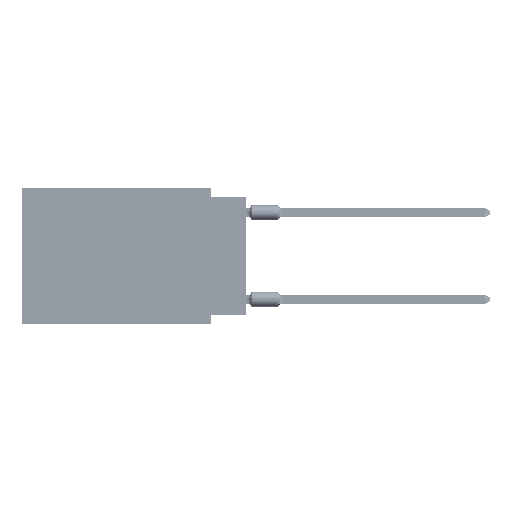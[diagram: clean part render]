
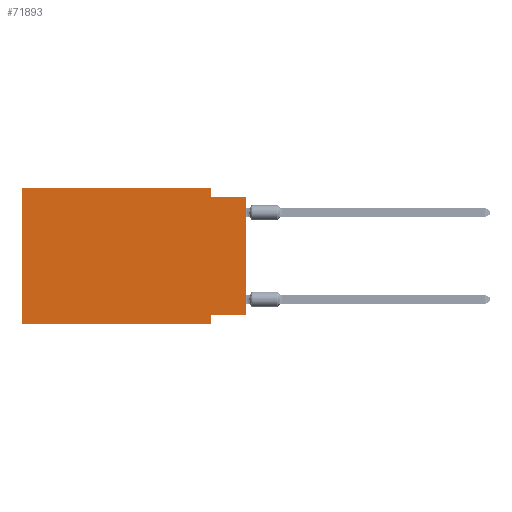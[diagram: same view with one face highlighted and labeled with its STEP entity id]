
A CAD part, left-side view. The second image highlights one B-rep face of the part: STEP entity #71893.
In plain terms, the highlighted planar face has unit normal (-1, 0, 0).
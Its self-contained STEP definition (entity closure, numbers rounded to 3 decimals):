
#214 = CARTESIAN_POINT ( 'NONE',  ( 0., 16.383, 0. ) ) ;
#407 = CARTESIAN_POINT ( 'NONE',  ( 0., 16.383, -9.906 ) ) ;
#1781 = LINE ( 'NONE', #71498, #9529 ) ;
#2015 = LINE ( 'NONE', #15659, #51012 ) ;
#5107 = EDGE_CURVE ( 'NONE', #33575, #48705, #1781, .T. ) ;
#5510 = CARTESIAN_POINT ( 'NONE',  ( 0., 16.383, 0. ) ) ;
#5823 = DIRECTION ( 'NONE',  ( 1., 0., 0. ) ) ;
#6408 = CARTESIAN_POINT ( 'NONE',  ( 0., 0., -0.635 ) ) ;
#9487 = DIRECTION ( 'NONE',  ( 0., 0., 1. ) ) ;
#9529 = VECTOR ( 'NONE', #23167, 1000. ) ;
#9564 = ORIENTED_EDGE ( 'NONE', *, *, #29825, .F. ) ;
#10591 = VERTEX_POINT ( 'NONE', #35574 ) ;
#11127 = VECTOR ( 'NONE', #9487, 1000. ) ;
#11436 = DIRECTION ( 'NONE',  ( 0., -1., 0. ) ) ;
#12645 = FACE_OUTER_BOUND ( 'NONE', #25397, .T. ) ;
#12924 = CARTESIAN_POINT ( 'NONE',  ( 0., 2.54, -9.906 ) ) ;
#15659 = CARTESIAN_POINT ( 'NONE',  ( 0., 0., -0.635 ) ) ;
#19621 = DIRECTION ( 'NONE',  ( 0., -1., 0. ) ) ;
#20076 = ORIENTED_EDGE ( 'NONE', *, *, #5107, .F. ) ;
#21809 = CARTESIAN_POINT ( 'NONE',  ( 0., 2.54, -9.271 ) ) ;
#22776 = EDGE_CURVE ( 'NONE', #80145, #86815, #71934, .T. ) ;
#23085 = CARTESIAN_POINT ( 'NONE',  ( 0., 0., -9.271 ) ) ;
#23167 = DIRECTION ( 'NONE',  ( 0., 0., -1. ) ) ;
#24443 = LINE ( 'NONE', #23085, #74344 ) ;
#25397 = EDGE_LOOP ( 'NONE', ( #33889, #69377, #9564, #27735, #79737, #35494, #20076, #78307 ) ) ;
#25433 = VECTOR ( 'NONE', #43156, 1000. ) ;
#27735 = ORIENTED_EDGE ( 'NONE', *, *, #51779, .F. ) ;
#29825 = EDGE_CURVE ( 'NONE', #10591, #76519, #44057, .T. ) ;
#31224 = VERTEX_POINT ( 'NONE', #407 ) ;
#31900 = VECTOR ( 'NONE', #11436, 1000. ) ;
#33575 = VERTEX_POINT ( 'NONE', #21809 ) ;
#33889 = ORIENTED_EDGE ( 'NONE', *, *, #22776, .T. ) ;
#33944 = AXIS2_PLACEMENT_3D ( 'NONE', #68262, #5823, #79807 ) ;
#35494 = ORIENTED_EDGE ( 'NONE', *, *, #82817, .T. ) ;
#35574 = CARTESIAN_POINT ( 'NONE',  ( 0., 2.54, 0. ) ) ;
#37668 = DIRECTION ( 'NONE',  ( 0., 1., 0. ) ) ;
#38788 = CARTESIAN_POINT ( 'NONE',  ( 0., 16.383, -9.906 ) ) ;
#40441 = PLANE ( 'NONE',  #33944 ) ;
#40640 = CARTESIAN_POINT ( 'NONE',  ( 0., 0., -9.271 ) ) ;
#43156 = DIRECTION ( 'NONE',  ( 0., 0., -1. ) ) ;
#44057 = LINE ( 'NONE', #85517, #25433 ) ;
#45671 = VECTOR ( 'NONE', #79933, 1000. ) ;
#48705 = VERTEX_POINT ( 'NONE', #12924 ) ;
#49818 = EDGE_CURVE ( 'NONE', #76519, #86815, #2015, .T. ) ;
#51012 = VECTOR ( 'NONE', #85384, 1000. ) ;
#51235 = LINE ( 'NONE', #86307, #45671 ) ;
#51779 = EDGE_CURVE ( 'NONE', #64633, #10591, #82512, .T. ) ;
#51879 = CARTESIAN_POINT ( 'NONE',  ( 0., 0., 0. ) ) ;
#58664 = CARTESIAN_POINT ( 'NONE',  ( 0., 2.54, -0.635 ) ) ;
#61483 = VECTOR ( 'NONE', #19621, 1000. ) ;
#64633 = VERTEX_POINT ( 'NONE', #214 ) ;
#67938 = EDGE_CURVE ( 'NONE', #80145, #33575, #24443, .T. ) ;
#68262 = CARTESIAN_POINT ( 'NONE',  ( 0., 16.383, 0. ) ) ;
#69377 = ORIENTED_EDGE ( 'NONE', *, *, #49818, .F. ) ;
#71498 = CARTESIAN_POINT ( 'NONE',  ( 0., 2.54, -9.906 ) ) ;
#71893 = ADVANCED_FACE ( 'NONE', ( #12645 ), #40441, .F. ) ;
#71934 = LINE ( 'NONE', #51879, #11127 ) ;
#72492 = EDGE_CURVE ( 'NONE', #31224, #64633, #51235, .T. ) ;
#73895 = LINE ( 'NONE', #38788, #31900 ) ;
#74344 = VECTOR ( 'NONE', #37668, 1000. ) ;
#76519 = VERTEX_POINT ( 'NONE', #58664 ) ;
#78307 = ORIENTED_EDGE ( 'NONE', *, *, #67938, .F. ) ;
#79737 = ORIENTED_EDGE ( 'NONE', *, *, #72492, .F. ) ;
#79807 = DIRECTION ( 'NONE',  ( 0., 0., -1. ) ) ;
#79933 = DIRECTION ( 'NONE',  ( 0., 0., 1. ) ) ;
#80145 = VERTEX_POINT ( 'NONE', #40640 ) ;
#82512 = LINE ( 'NONE', #5510, #61483 ) ;
#82817 = EDGE_CURVE ( 'NONE', #31224, #48705, #73895, .T. ) ;
#85384 = DIRECTION ( 'NONE',  ( 0., -1., 0. ) ) ;
#85517 = CARTESIAN_POINT ( 'NONE',  ( 0., 2.54, 0. ) ) ;
#86307 = CARTESIAN_POINT ( 'NONE',  ( 0., 16.383, 0. ) ) ;
#86815 = VERTEX_POINT ( 'NONE', #6408 ) ;
